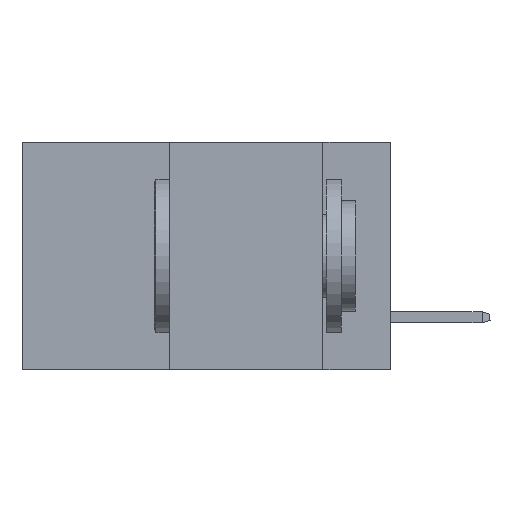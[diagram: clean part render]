
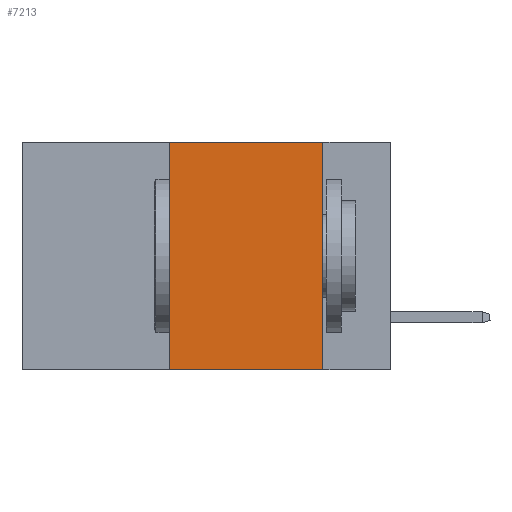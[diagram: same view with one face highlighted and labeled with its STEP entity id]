
A CAD part, left-side view. The second image highlights one B-rep face of the part: STEP entity #7213.
In plain terms, the highlighted planar face has unit normal (-1, 0, 0).
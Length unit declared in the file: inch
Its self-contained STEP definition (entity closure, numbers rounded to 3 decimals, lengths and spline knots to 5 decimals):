
#279 = CARTESIAN_POINT ( 'NONE',  ( 0., 0.11, -0.37 ) ) ;
#281 = VECTOR ( 'NONE', #4020, 39.37008 ) ;
#635 = EDGE_CURVE ( 'NONE', #1394, #6900, #4937, .T. ) ;
#960 = VECTOR ( 'NONE', #3519, 39.37008 ) ;
#1031 = ORIENTED_EDGE ( 'NONE', *, *, #7707, .F. ) ;
#1394 = VERTEX_POINT ( 'NONE', #7715 ) ;
#1659 = EDGE_CURVE ( 'NONE', #8358, #6535, #7440, .T. ) ;
#1695 = CARTESIAN_POINT ( 'NONE',  ( 0., 0.11, 0. ) ) ;
#1973 = AXIS2_PLACEMENT_3D ( 'NONE', #3016, #4477, #5228 ) ;
#3016 = CARTESIAN_POINT ( 'NONE',  ( 0., 0.6, 0. ) ) ;
#3334 = VECTOR ( 'NONE', #9117, 39.37008 ) ;
#3519 = DIRECTION ( 'NONE',  ( 0., -1., 0. ) ) ;
#4020 = DIRECTION ( 'NONE',  ( 0., 0., -1. ) ) ;
#4119 = VECTOR ( 'NONE', #5075, 39.37008 ) ;
#4477 = DIRECTION ( 'NONE',  ( 1., 0., 0. ) ) ;
#4513 = EDGE_CURVE ( 'NONE', #1394, #8358, #5543, .T. ) ;
#4817 = PLANE ( 'NONE',  #1973 ) ;
#4886 = ORIENTED_EDGE ( 'NONE', *, *, #635, .T. ) ;
#4937 = LINE ( 'NONE', #9508, #4119 ) ;
#5075 = DIRECTION ( 'NONE',  ( 0., -1., 0. ) ) ;
#5228 = DIRECTION ( 'NONE',  ( 0., 0., -1. ) ) ;
#5357 = EDGE_LOOP ( 'NONE', ( #1031, #8011, #7505, #4886 ) ) ;
#5512 = FACE_OUTER_BOUND ( 'NONE', #5357, .T. ) ;
#5543 = LINE ( 'NONE', #8368, #3334 ) ;
#5746 = CARTESIAN_POINT ( 'NONE',  ( 0., 0.6, 0. ) ) ;
#6535 = VERTEX_POINT ( 'NONE', #9133 ) ;
#6900 = VERTEX_POINT ( 'NONE', #279 ) ;
#7213 = ADVANCED_FACE ( 'NONE', ( #5512 ), #4817, .F. ) ;
#7440 = LINE ( 'NONE', #5746, #960 ) ;
#7505 = ORIENTED_EDGE ( 'NONE', *, *, #4513, .F. ) ;
#7698 = LINE ( 'NONE', #1695, #281 ) ;
#7707 = EDGE_CURVE ( 'NONE', #6535, #6900, #7698, .T. ) ;
#7715 = CARTESIAN_POINT ( 'NONE',  ( 0., 0.36, -0.37 ) ) ;
#8011 = ORIENTED_EDGE ( 'NONE', *, *, #1659, .F. ) ;
#8358 = VERTEX_POINT ( 'NONE', #8878 ) ;
#8368 = CARTESIAN_POINT ( 'NONE',  ( 0., 0.36, 0. ) ) ;
#8878 = CARTESIAN_POINT ( 'NONE',  ( 0., 0.36, 0. ) ) ;
#9117 = DIRECTION ( 'NONE',  ( 0., 0., 1. ) ) ;
#9133 = CARTESIAN_POINT ( 'NONE',  ( 0., 0.11, 0. ) ) ;
#9508 = CARTESIAN_POINT ( 'NONE',  ( 0., 0.6, -0.37 ) ) ;
